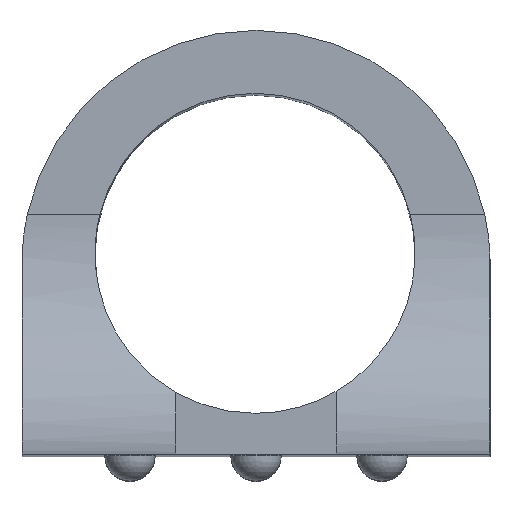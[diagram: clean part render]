
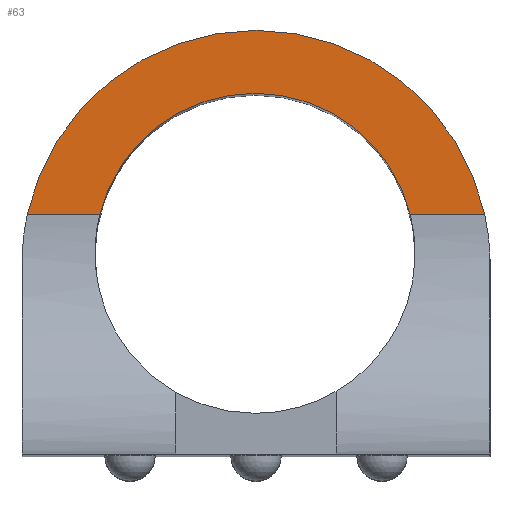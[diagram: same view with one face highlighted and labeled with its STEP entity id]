
A CAD part, top view. The second image highlights one B-rep face of the part: STEP entity #63.
In plain terms, the highlighted planar face has unit normal (0, 0, 1).
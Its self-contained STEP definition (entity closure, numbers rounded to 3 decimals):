
#13 = VERTEX_POINT ( 'NONE', #940 ) ;
#63 = ADVANCED_FACE ( 'NONE', ( #575 ), #509, .T. ) ;
#66 = CARTESIAN_POINT ( 'NONE',  ( 44.058, 43.328, -15.408 ) ) ;
#87 = DIRECTION ( 'NONE',  ( 1., 0., 0. ) ) ;
#88 = DIRECTION ( 'NONE',  ( 0., 0., -1. ) ) ;
#89 = CARTESIAN_POINT ( 'NONE',  ( 31.739, 40.242, -15.408 ) ) ;
#106 = AXIS2_PLACEMENT_3D ( 'NONE', #89, #88, #87 ) ;
#130 = CIRCLE ( 'NONE', #106, 12.7 ) ;
#199 = CIRCLE ( 'NONE', #268, 18.575 ) ;
#213 = EDGE_CURVE ( 'NONE', #13, #989, #501, .T. ) ;
#252 = DIRECTION ( 'NONE',  ( 1., 0., 0. ) ) ;
#255 = DIRECTION ( 'NONE',  ( 0., 0., 1. ) ) ;
#257 = CARTESIAN_POINT ( 'NONE',  ( 31.815, 39.361, -15.408 ) ) ;
#268 = AXIS2_PLACEMENT_3D ( 'NONE', #257, #255, #252 ) ;
#337 = CARTESIAN_POINT ( 'NONE',  ( 31.739, 52.942, -15.408 ) ) ;
#421 = VECTOR ( 'NONE', #857, 1000. ) ;
#443 = LINE ( 'NONE', #860, #421 ) ;
#477 = DIRECTION ( 'NONE',  ( 1., 0., 0. ) ) ;
#484 = CIRCLE ( 'NONE', #582, 12.7 ) ;
#497 = VECTOR ( 'NONE', #1277, 1000. ) ;
#499 = DIRECTION ( 'NONE',  ( 0., 0., 1. ) ) ;
#501 = LINE ( 'NONE', #1278, #497 ) ;
#509 = PLANE ( 'NONE',  #807 ) ;
#538 = CARTESIAN_POINT ( 'NONE',  ( 50.382, 17.915, -15.408 ) ) ;
#573 = EDGE_CURVE ( 'NONE', #13, #1126, #484, .T. ) ;
#575 = FACE_OUTER_BOUND ( 'NONE', #786, .T. ) ;
#582 = AXIS2_PLACEMENT_3D ( 'NONE', #1061, #1059, #1056 ) ;
#705 = VERTEX_POINT ( 'NONE', #1077 ) ;
#754 = CARTESIAN_POINT ( 'NONE',  ( 13.668, 43.328, -15.408 ) ) ;
#786 = EDGE_LOOP ( 'NONE', ( #1060, #1062, #1066, #1068, #1070 ) ) ;
#807 = AXIS2_PLACEMENT_3D ( 'NONE', #538, #499, #477 ) ;
#857 = DIRECTION ( 'NONE',  ( -1., 0., 0. ) ) ;
#860 = CARTESIAN_POINT ( 'NONE',  ( 50.281, 43.328, -15.408 ) ) ;
#940 = CARTESIAN_POINT ( 'NONE',  ( 19.419, 43.328, -15.408 ) ) ;
#972 = EDGE_CURVE ( 'NONE', #705, #1312, #443, .T. ) ;
#989 = VERTEX_POINT ( 'NONE', #754 ) ;
#1056 = DIRECTION ( 'NONE',  ( 1., 0., 0. ) ) ;
#1059 = DIRECTION ( 'NONE',  ( 0., 0., -1. ) ) ;
#1060 = ORIENTED_EDGE ( 'NONE', *, *, #972, .F. ) ;
#1061 = CARTESIAN_POINT ( 'NONE',  ( 31.739, 40.242, -15.408 ) ) ;
#1062 = ORIENTED_EDGE ( 'NONE', *, *, #1192, .T. ) ;
#1066 = ORIENTED_EDGE ( 'NONE', *, *, #213, .F. ) ;
#1068 = ORIENTED_EDGE ( 'NONE', *, *, #573, .T. ) ;
#1070 = ORIENTED_EDGE ( 'NONE', *, *, #1295, .T. ) ;
#1077 = CARTESIAN_POINT ( 'NONE',  ( 49.961, 43.328, -15.408 ) ) ;
#1126 = VERTEX_POINT ( 'NONE', #337 ) ;
#1192 = EDGE_CURVE ( 'NONE', #705, #989, #199, .T. ) ;
#1277 = DIRECTION ( 'NONE',  ( -1., 0., 0. ) ) ;
#1278 = CARTESIAN_POINT ( 'NONE',  ( 50.281, 43.328, -15.408 ) ) ;
#1295 = EDGE_CURVE ( 'NONE', #1126, #1312, #130, .T. ) ;
#1312 = VERTEX_POINT ( 'NONE', #66 ) ;
